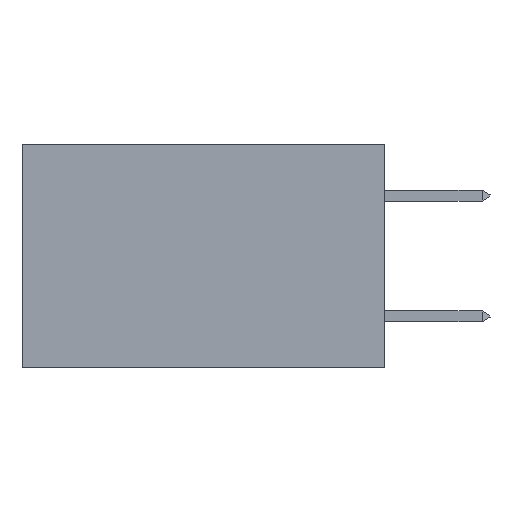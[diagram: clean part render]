
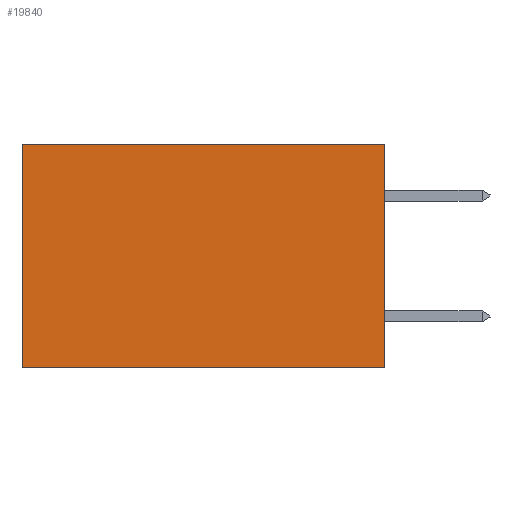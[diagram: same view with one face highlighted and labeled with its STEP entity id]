
A CAD part, left-side view. The second image highlights one B-rep face of the part: STEP entity #19840.
In plain terms, the highlighted planar face has unit normal (-1, 0, 0).
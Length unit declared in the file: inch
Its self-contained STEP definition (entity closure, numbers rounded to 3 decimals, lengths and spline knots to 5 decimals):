
#225 = DIRECTION ( 'NONE',  ( 1., 0., 0. ) ) ;
#1831 = CARTESIAN_POINT ( 'NONE',  ( 0.2875, 0., 0. ) ) ;
#1833 = LINE ( 'NONE', #21303, #10942 ) ;
#2702 = EDGE_CURVE ( 'NONE', #30204, #8307, #27637, .T. ) ;
#3545 = CARTESIAN_POINT ( 'NONE',  ( 0.2875, 0.6, -0.37 ) ) ;
#3637 = CARTESIAN_POINT ( 'NONE',  ( 0.2875, 0., 0. ) ) ;
#5791 = PLANE ( 'NONE',  #18600 ) ;
#5929 = LINE ( 'NONE', #3637, #28484 ) ;
#5980 = DIRECTION ( 'NONE',  ( 0., 1., 0. ) ) ;
#6967 = ORIENTED_EDGE ( 'NONE', *, *, #28670, .F. ) ;
#8307 = VERTEX_POINT ( 'NONE', #3545 ) ;
#10575 = EDGE_LOOP ( 'NONE', ( #17347, #6967, #13764, #17979 ) ) ;
#10942 = VECTOR ( 'NONE', #14181, 39.37008 ) ;
#13764 = ORIENTED_EDGE ( 'NONE', *, *, #23314, .F. ) ;
#14181 = DIRECTION ( 'NONE',  ( 0., 1., 0. ) ) ;
#14797 = LINE ( 'NONE', #1831, #19942 ) ;
#16049 = CARTESIAN_POINT ( 'NONE',  ( 0.2875, 0.6, 0. ) ) ;
#16274 = VECTOR ( 'NONE', #25418, 39.37008 ) ;
#16291 = DIRECTION ( 'NONE',  ( 0., 0., -1. ) ) ;
#17047 = EDGE_CURVE ( 'NONE', #22881, #30204, #5929, .T. ) ;
#17347 = ORIENTED_EDGE ( 'NONE', *, *, #2702, .T. ) ;
#17979 = ORIENTED_EDGE ( 'NONE', *, *, #17047, .T. ) ;
#18600 = AXIS2_PLACEMENT_3D ( 'NONE', #28697, #225, #16291 ) ;
#19681 = CARTESIAN_POINT ( 'NONE',  ( 0.2875, 0.6, 0. ) ) ;
#19840 = ADVANCED_FACE ( 'NONE', ( #27975 ), #5791, .F. ) ;
#19942 = VECTOR ( 'NONE', #25144, 39.37008 ) ;
#21303 = CARTESIAN_POINT ( 'NONE',  ( 0.2875, 0., -0.37 ) ) ;
#22356 = CARTESIAN_POINT ( 'NONE',  ( 0.2875, 0., -0.37 ) ) ;
#22648 = VERTEX_POINT ( 'NONE', #22356 ) ;
#22881 = VERTEX_POINT ( 'NONE', #23534 ) ;
#23314 = EDGE_CURVE ( 'NONE', #22881, #22648, #14797, .T. ) ;
#23534 = CARTESIAN_POINT ( 'NONE',  ( 0.2875, 0., 0. ) ) ;
#25144 = DIRECTION ( 'NONE',  ( 0., 0., -1. ) ) ;
#25418 = DIRECTION ( 'NONE',  ( 0., 0., -1. ) ) ;
#27637 = LINE ( 'NONE', #16049, #16274 ) ;
#27975 = FACE_OUTER_BOUND ( 'NONE', #10575, .T. ) ;
#28484 = VECTOR ( 'NONE', #5980, 39.37008 ) ;
#28670 = EDGE_CURVE ( 'NONE', #22648, #8307, #1833, .T. ) ;
#28697 = CARTESIAN_POINT ( 'NONE',  ( 0.2875, 0., 0. ) ) ;
#30204 = VERTEX_POINT ( 'NONE', #19681 ) ;
